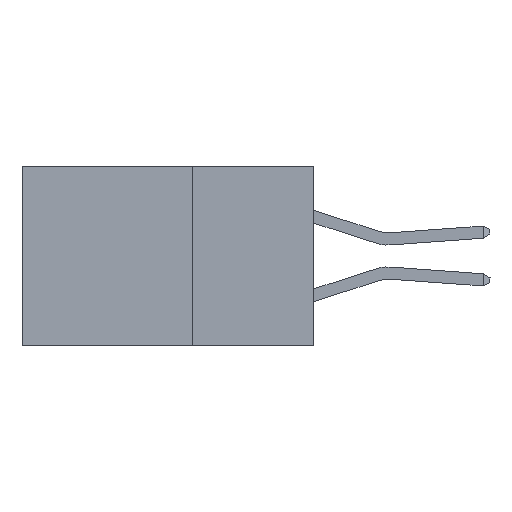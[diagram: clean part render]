
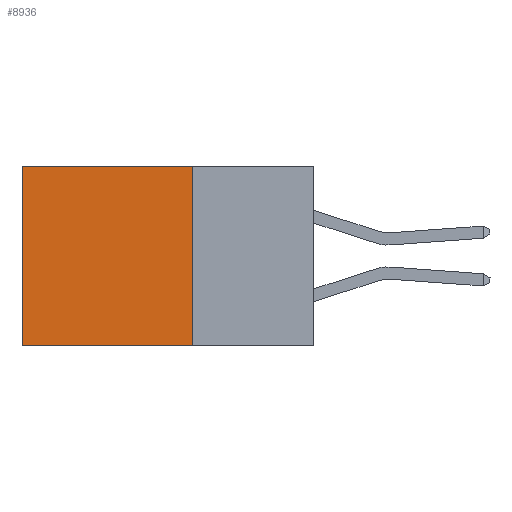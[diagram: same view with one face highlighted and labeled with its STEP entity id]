
A CAD part, left-side view. The second image highlights one B-rep face of the part: STEP entity #8936.
In plain terms, the highlighted planar face has unit normal (-1, 0, 0).
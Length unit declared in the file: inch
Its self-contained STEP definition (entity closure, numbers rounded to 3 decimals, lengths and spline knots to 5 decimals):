
#583 = EDGE_LOOP ( 'NONE', ( #32630, #21494, #29411, #22874 ) ) ;
#1186 = CARTESIAN_POINT ( 'NONE',  ( 0.2875, 0.25, 0. ) ) ;
#2750 = VERTEX_POINT ( 'NONE', #8848 ) ;
#3256 = VECTOR ( 'NONE', #3852, 39.37008 ) ;
#3852 = DIRECTION ( 'NONE',  ( 0., 1., 0. ) ) ;
#4311 = VERTEX_POINT ( 'NONE', #6784 ) ;
#4684 = PLANE ( 'NONE',  #29849 ) ;
#5327 = LINE ( 'NONE', #14009, #25285 ) ;
#6211 = EDGE_CURVE ( 'NONE', #24332, #2750, #5327, .T. ) ;
#6784 = CARTESIAN_POINT ( 'NONE',  ( 0.2875, 0.25, -0.37 ) ) ;
#7113 = CARTESIAN_POINT ( 'NONE',  ( 0.2875, 0.6, 0. ) ) ;
#7275 = DIRECTION ( 'NONE',  ( 1., 0., 0. ) ) ;
#8848 = CARTESIAN_POINT ( 'NONE',  ( 0.2875, 0.6, -0.37 ) ) ;
#8936 = ADVANCED_FACE ( 'NONE', ( #22677 ), #4684, .F. ) ;
#9868 = DIRECTION ( 'NONE',  ( 0., 0., -1. ) ) ;
#11382 = LINE ( 'NONE', #21861, #3256 ) ;
#11896 = DIRECTION ( 'NONE',  ( 0., 1., 0. ) ) ;
#14009 = CARTESIAN_POINT ( 'NONE',  ( 0.2875, 0.6, 0. ) ) ;
#15427 = VERTEX_POINT ( 'NONE', #1186 ) ;
#20641 = EDGE_CURVE ( 'NONE', #4311, #2750, #11382, .T. ) ;
#21494 = ORIENTED_EDGE ( 'NONE', *, *, #20641, .F. ) ;
#21682 = VECTOR ( 'NONE', #31127, 39.37008 ) ;
#21861 = CARTESIAN_POINT ( 'NONE',  ( 0.2875, 0.25, -0.37 ) ) ;
#22677 = FACE_OUTER_BOUND ( 'NONE', #583, .T. ) ;
#22874 = ORIENTED_EDGE ( 'NONE', *, *, #31585, .T. ) ;
#23252 = VECTOR ( 'NONE', #11896, 39.37008 ) ;
#23310 = LINE ( 'NONE', #28715, #21682 ) ;
#24332 = VERTEX_POINT ( 'NONE', #7113 ) ;
#25285 = VECTOR ( 'NONE', #26661, 39.37008 ) ;
#26661 = DIRECTION ( 'NONE',  ( 0., 0., -1. ) ) ;
#27745 = CARTESIAN_POINT ( 'NONE',  ( 0.2875, 0.25, 0. ) ) ;
#28715 = CARTESIAN_POINT ( 'NONE',  ( 0.2875, 0.25, 0. ) ) ;
#28910 = LINE ( 'NONE', #27745, #23252 ) ;
#29411 = ORIENTED_EDGE ( 'NONE', *, *, #30595, .F. ) ;
#29849 = AXIS2_PLACEMENT_3D ( 'NONE', #30531, #7275, #9868 ) ;
#30531 = CARTESIAN_POINT ( 'NONE',  ( 0.2875, 0.25, 0. ) ) ;
#30595 = EDGE_CURVE ( 'NONE', #15427, #4311, #23310, .T. ) ;
#31127 = DIRECTION ( 'NONE',  ( 0., 0., -1. ) ) ;
#31585 = EDGE_CURVE ( 'NONE', #15427, #24332, #28910, .T. ) ;
#32630 = ORIENTED_EDGE ( 'NONE', *, *, #6211, .T. ) ;
